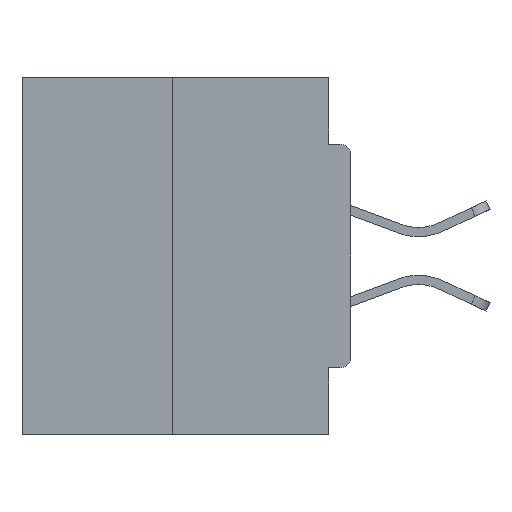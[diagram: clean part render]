
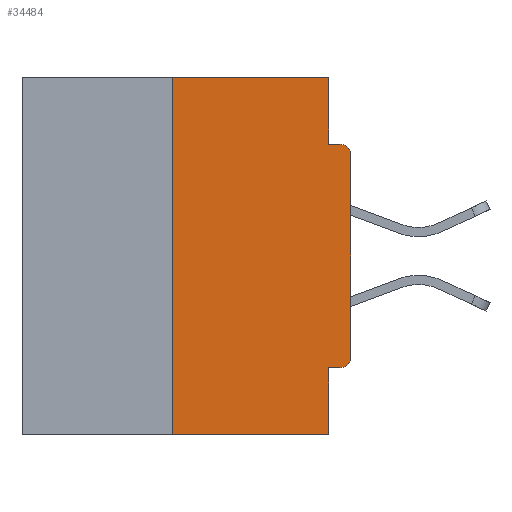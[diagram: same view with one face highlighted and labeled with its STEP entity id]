
A CAD part, left-side view. The second image highlights one B-rep face of the part: STEP entity #34484.
In plain terms, the highlighted planar face has unit normal (-1, 0, 0).
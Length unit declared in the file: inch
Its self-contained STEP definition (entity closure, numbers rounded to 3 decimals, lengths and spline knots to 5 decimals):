
#570 = CARTESIAN_POINT ( 'NONE',  ( 0., 0.031, -0.5 ) ) ;
#2251 = DIRECTION ( 'NONE',  ( 0., 0., -1. ) ) ;
#2252 = CARTESIAN_POINT ( 'NONE',  ( 0., 0.015, -0.1085 ) ) ;
#2635 = LINE ( 'NONE', #28167, #14285 ) ;
#3304 = VERTEX_POINT ( 'NONE', #29996 ) ;
#3712 = CARTESIAN_POINT ( 'NONE',  ( 0., 0.46, 0. ) ) ;
#4545 = ORIENTED_EDGE ( 'NONE', *, *, #24553, .T. ) ;
#4613 = ORIENTED_EDGE ( 'NONE', *, *, #18277, .F. ) ;
#4742 = CARTESIAN_POINT ( 'NONE',  ( 0., 0., -0.3915 ) ) ;
#4926 = LINE ( 'NONE', #21023, #22365 ) ;
#5383 = EDGE_CURVE ( 'NONE', #13766, #24087, #37366, .T. ) ;
#6396 = EDGE_CURVE ( 'NONE', #21873, #28468, #9995, .T. ) ;
#6514 = DIRECTION ( 'NONE',  ( 0., 0., 1. ) ) ;
#6877 = CARTESIAN_POINT ( 'NONE',  ( 0., 0.031, 0. ) ) ;
#6878 = VECTOR ( 'NONE', #8709, 39.37008 ) ;
#7466 = LINE ( 'NONE', #570, #24887 ) ;
#7884 = ORIENTED_EDGE ( 'NONE', *, *, #19761, .F. ) ;
#8289 = VECTOR ( 'NONE', #29259, 39.37008 ) ;
#8493 = CARTESIAN_POINT ( 'NONE',  ( 0., 0.25, 0. ) ) ;
#8529 = DIRECTION ( 'NONE',  ( 0., 0., -1. ) ) ;
#8602 = CARTESIAN_POINT ( 'NONE',  ( 0., 0.031, 0. ) ) ;
#8709 = DIRECTION ( 'NONE',  ( 0., 1., 0. ) ) ;
#8765 = LINE ( 'NONE', #14873, #28346 ) ;
#9341 = FACE_OUTER_BOUND ( 'NONE', #15146, .T. ) ;
#9424 = CARTESIAN_POINT ( 'NONE',  ( 0., 0., 0. ) ) ;
#9672 = VERTEX_POINT ( 'NONE', #18652 ) ;
#9688 = VERTEX_POINT ( 'NONE', #8493 ) ;
#9995 = LINE ( 'NONE', #6877, #8289 ) ;
#10694 = CARTESIAN_POINT ( 'NONE',  ( 0., 0.015, -0.4065 ) ) ;
#11682 = CARTESIAN_POINT ( 'NONE',  ( 0., 0., -0.4065 ) ) ;
#12694 = CARTESIAN_POINT ( 'NONE',  ( 0., 0.031, -0.4065 ) ) ;
#13156 = DIRECTION ( 'NONE',  ( 0., 0., -1. ) ) ;
#13544 = DIRECTION ( 'NONE',  ( 0., 0., -1. ) ) ;
#13766 = VERTEX_POINT ( 'NONE', #10694 ) ;
#14285 = VECTOR ( 'NONE', #40916, 39.37008 ) ;
#14873 = CARTESIAN_POINT ( 'NONE',  ( 0., 0.25, 0. ) ) ;
#15146 = EDGE_LOOP ( 'NONE', ( #7884, #21581, #21198, #28579, #22411, #20984, #4545, #17204, #4613, #31986 ) ) ;
#17204 = ORIENTED_EDGE ( 'NONE', *, *, #19279, .T. ) ;
#17429 = EDGE_CURVE ( 'NONE', #24087, #9672, #7466, .T. ) ;
#17900 = DIRECTION ( 'NONE',  ( 0., -1., 0. ) ) ;
#18277 = EDGE_CURVE ( 'NONE', #28468, #31756, #2635, .T. ) ;
#18652 = CARTESIAN_POINT ( 'NONE',  ( 0., 0.031, -0.5 ) ) ;
#18842 = LINE ( 'NONE', #9424, #37009 ) ;
#19279 = EDGE_CURVE ( 'NONE', #3304, #31756, #38341, .T. ) ;
#19413 = DIRECTION ( 'NONE',  ( 0., -1., 0. ) ) ;
#19638 = LINE ( 'NONE', #37858, #38757 ) ;
#19761 = EDGE_CURVE ( 'NONE', #9688, #21873, #4926, .T. ) ;
#20984 = ORIENTED_EDGE ( 'NONE', *, *, #24007, .T. ) ;
#21023 = CARTESIAN_POINT ( 'NONE',  ( 0., 0.46, 0. ) ) ;
#21198 = ORIENTED_EDGE ( 'NONE', *, *, #29218, .T. ) ;
#21581 = ORIENTED_EDGE ( 'NONE', *, *, #24828, .F. ) ;
#21645 = AXIS2_PLACEMENT_3D ( 'NONE', #2252, #40539, #8529 ) ;
#21873 = VERTEX_POINT ( 'NONE', #8602 ) ;
#22085 = PLANE ( 'NONE',  #40369 ) ;
#22365 = VECTOR ( 'NONE', #17900, 39.37008 ) ;
#22411 = ORIENTED_EDGE ( 'NONE', *, *, #5383, .F. ) ;
#22701 = CARTESIAN_POINT ( 'NONE',  ( 0., 0.031, -0.0935 ) ) ;
#23303 = VERTEX_POINT ( 'NONE', #25314 ) ;
#23577 = CIRCLE ( 'NONE', #24231, 0.015 ) ;
#23932 = VERTEX_POINT ( 'NONE', #4742 ) ;
#24007 = EDGE_CURVE ( 'NONE', #13766, #23932, #23577, .T. ) ;
#24087 = VERTEX_POINT ( 'NONE', #12694 ) ;
#24231 = AXIS2_PLACEMENT_3D ( 'NONE', #30907, #40537, #2251 ) ;
#24553 = EDGE_CURVE ( 'NONE', #23932, #3304, #18842, .T. ) ;
#24828 = EDGE_CURVE ( 'NONE', #23303, #9688, #8765, .T. ) ;
#24887 = VECTOR ( 'NONE', #13156, 39.37008 ) ;
#25314 = CARTESIAN_POINT ( 'NONE',  ( 0., 0.25, -0.5 ) ) ;
#25671 = DIRECTION ( 'NONE',  ( 1., 0., 0. ) ) ;
#28167 = CARTESIAN_POINT ( 'NONE',  ( 0., 0., -0.0935 ) ) ;
#28346 = VECTOR ( 'NONE', #36793, 39.37008 ) ;
#28468 = VERTEX_POINT ( 'NONE', #22701 ) ;
#28579 = ORIENTED_EDGE ( 'NONE', *, *, #17429, .F. ) ;
#29218 = EDGE_CURVE ( 'NONE', #23303, #9672, #19638, .T. ) ;
#29259 = DIRECTION ( 'NONE',  ( 0., 0., -1. ) ) ;
#29996 = CARTESIAN_POINT ( 'NONE',  ( 0., 0., -0.1085 ) ) ;
#30907 = CARTESIAN_POINT ( 'NONE',  ( 0., 0.015, -0.3915 ) ) ;
#31756 = VERTEX_POINT ( 'NONE', #34949 ) ;
#31986 = ORIENTED_EDGE ( 'NONE', *, *, #6396, .F. ) ;
#34484 = ADVANCED_FACE ( 'NONE', ( #9341 ), #22085, .F. ) ;
#34949 = CARTESIAN_POINT ( 'NONE',  ( 0., 0.015, -0.0935 ) ) ;
#36793 = DIRECTION ( 'NONE',  ( 0., 0., 1. ) ) ;
#37009 = VECTOR ( 'NONE', #6514, 39.37008 ) ;
#37366 = LINE ( 'NONE', #11682, #6878 ) ;
#37858 = CARTESIAN_POINT ( 'NONE',  ( 0., 0.46, -0.5 ) ) ;
#38341 = CIRCLE ( 'NONE', #21645, 0.015 ) ;
#38757 = VECTOR ( 'NONE', #19413, 39.37008 ) ;
#40369 = AXIS2_PLACEMENT_3D ( 'NONE', #3712, #25671, #13544 ) ;
#40537 = DIRECTION ( 'NONE',  ( -1., 0., 0. ) ) ;
#40539 = DIRECTION ( 'NONE',  ( -1., 0., 0. ) ) ;
#40916 = DIRECTION ( 'NONE',  ( 0., -1., 0. ) ) ;
